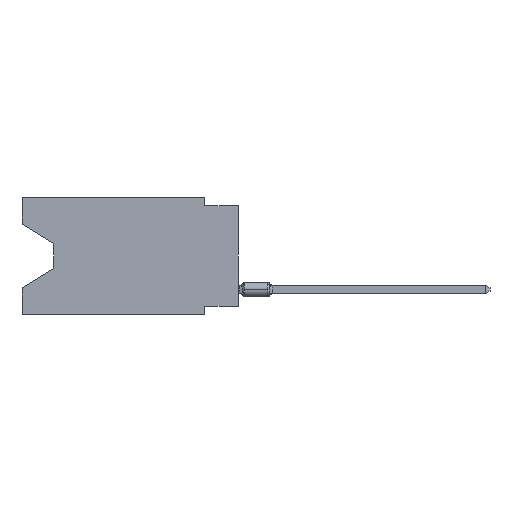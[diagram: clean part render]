
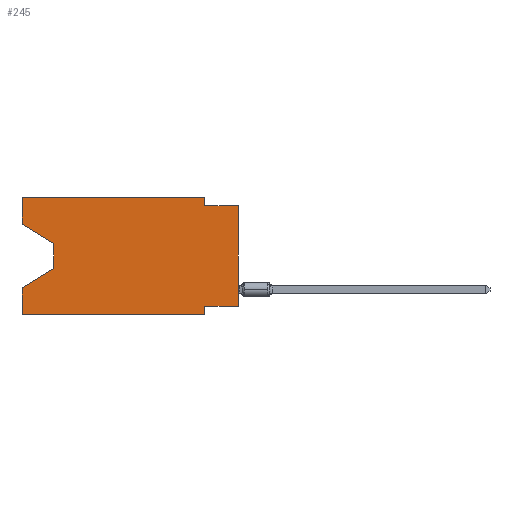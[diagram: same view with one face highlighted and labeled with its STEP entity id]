
A CAD part, left-side view. The second image highlights one B-rep face of the part: STEP entity #245.
In plain terms, the highlighted planar face has unit normal (-1, 0, 0).
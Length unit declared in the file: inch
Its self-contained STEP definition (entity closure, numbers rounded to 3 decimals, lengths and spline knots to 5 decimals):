
#217 = VERTEX_POINT ( 'NONE', #4701 ) ;
#245 = ADVANCED_FACE ( 'NONE', ( #24458 ), #6535, .F. ) ;
#332 = CARTESIAN_POINT ( 'NONE',  ( 0., 0.55, -0.212 ) ) ;
#547 = DIRECTION ( 'NONE',  ( 0., 0., -1. ) ) ;
#1364 = VECTOR ( 'NONE', #547, 39.37008 ) ;
#2369 = DIRECTION ( 'NONE',  ( 0., 0., -1. ) ) ;
#2490 = CARTESIAN_POINT ( 'NONE',  ( 0., 0.1, 0. ) ) ;
#2814 = CARTESIAN_POINT ( 'NONE',  ( 0., 0.645, -0.08025 ) ) ;
#3760 = ORIENTED_EDGE ( 'NONE', *, *, #13887, .T. ) ;
#3884 = LINE ( 'NONE', #23644, #7617 ) ;
#4409 = LINE ( 'NONE', #12259, #15118 ) ;
#4701 = CARTESIAN_POINT ( 'NONE',  ( 0., 0.1, -0.025 ) ) ;
#5200 = LINE ( 'NONE', #8858, #8436 ) ;
#5216 = ORIENTED_EDGE ( 'NONE', *, *, #17313, .F. ) ;
#5710 = DIRECTION ( 'NONE',  ( 0., -1., 0. ) ) ;
#6052 = DIRECTION ( 'NONE',  ( 0., 0., 1. ) ) ;
#6139 = CARTESIAN_POINT ( 'NONE',  ( 0., 0.55, -0.138 ) ) ;
#6485 = VERTEX_POINT ( 'NONE', #6589 ) ;
#6535 = PLANE ( 'NONE',  #13094 ) ;
#6589 = CARTESIAN_POINT ( 'NONE',  ( 0., 0.1, -0.35 ) ) ;
#6834 = VERTEX_POINT ( 'NONE', #2490 ) ;
#7025 = LINE ( 'NONE', #16592, #18294 ) ;
#7617 = VECTOR ( 'NONE', #5710, 39.37008 ) ;
#7631 = VERTEX_POINT ( 'NONE', #20921 ) ;
#7805 = DIRECTION ( 'NONE',  ( 0., 1., 0. ) ) ;
#8436 = VECTOR ( 'NONE', #18684, 39.37008 ) ;
#8643 = VECTOR ( 'NONE', #2369, 39.37008 ) ;
#8858 = CARTESIAN_POINT ( 'NONE',  ( 0., 0.645, 0. ) ) ;
#8985 = CARTESIAN_POINT ( 'NONE',  ( 0., 0.645, 0. ) ) ;
#9284 = EDGE_CURVE ( 'NONE', #16652, #6485, #23923, .T. ) ;
#9373 = ORIENTED_EDGE ( 'NONE', *, *, #17499, .T. ) ;
#9759 = CARTESIAN_POINT ( 'NONE',  ( 0., 0., -0.325 ) ) ;
#9935 = LINE ( 'NONE', #20303, #8643 ) ;
#10164 = CARTESIAN_POINT ( 'NONE',  ( 0., 0.645, -0.35 ) ) ;
#10638 = ORIENTED_EDGE ( 'NONE', *, *, #12898, .F. ) ;
#11161 = ORIENTED_EDGE ( 'NONE', *, *, #24345, .F. ) ;
#11797 = VERTEX_POINT ( 'NONE', #6139 ) ;
#11933 = EDGE_CURVE ( 'NONE', #16652, #7631, #5200, .T. ) ;
#12009 = EDGE_CURVE ( 'NONE', #25308, #6834, #3884, .T. ) ;
#12259 = CARTESIAN_POINT ( 'NONE',  ( 0., 0., 0. ) ) ;
#12898 = EDGE_CURVE ( 'NONE', #15807, #25308, #20046, .T. ) ;
#13094 = AXIS2_PLACEMENT_3D ( 'NONE', #20532, #20670, #14632 ) ;
#13154 = LINE ( 'NONE', #2814, #22991 ) ;
#13517 = VECTOR ( 'NONE', #22338, 39.37008 ) ;
#13703 = LINE ( 'NONE', #9759, #16769 ) ;
#13887 = EDGE_CURVE ( 'NONE', #15807, #11797, #13154, .T. ) ;
#14145 = ORIENTED_EDGE ( 'NONE', *, *, #17354, .F. ) ;
#14245 = DIRECTION ( 'NONE',  ( 0., -1., 0. ) ) ;
#14297 = DIRECTION ( 'NONE',  ( 0., -1., 0. ) ) ;
#14357 = LINE ( 'NONE', #22453, #13517 ) ;
#14573 = ORIENTED_EDGE ( 'NONE', *, *, #11933, .F. ) ;
#14632 = DIRECTION ( 'NONE',  ( 0., 0., -1. ) ) ;
#15118 = VECTOR ( 'NONE', #15911, 39.37008 ) ;
#15290 = ORIENTED_EDGE ( 'NONE', *, *, #23583, .T. ) ;
#15747 = EDGE_CURVE ( 'NONE', #11797, #22293, #16263, .T. ) ;
#15807 = VERTEX_POINT ( 'NONE', #20569 ) ;
#15911 = DIRECTION ( 'NONE',  ( 0., 0., 1. ) ) ;
#16263 = LINE ( 'NONE', #24106, #1364 ) ;
#16431 = VECTOR ( 'NONE', #6052, 39.37008 ) ;
#16592 = CARTESIAN_POINT ( 'NONE',  ( 0., 0.1, 0. ) ) ;
#16652 = VERTEX_POINT ( 'NONE', #10164 ) ;
#16745 = CARTESIAN_POINT ( 'NONE',  ( 0., 0., -0.025 ) ) ;
#16769 = VECTOR ( 'NONE', #7805, 39.37008 ) ;
#16840 = ORIENTED_EDGE ( 'NONE', *, *, #15747, .T. ) ;
#17313 = EDGE_CURVE ( 'NONE', #217, #17632, #24226, .T. ) ;
#17354 = EDGE_CURVE ( 'NONE', #24927, #23276, #13703, .T. ) ;
#17499 = EDGE_CURVE ( 'NONE', #24927, #17632, #4409, .T. ) ;
#17632 = VERTEX_POINT ( 'NONE', #19050 ) ;
#17650 = ORIENTED_EDGE ( 'NONE', *, *, #25441, .F. ) ;
#18294 = VECTOR ( 'NONE', #20521, 39.37008 ) ;
#18684 = DIRECTION ( 'NONE',  ( 0., 0., 1. ) ) ;
#19050 = CARTESIAN_POINT ( 'NONE',  ( 0., 0., -0.025 ) ) ;
#20046 = LINE ( 'NONE', #22015, #16431 ) ;
#20303 = CARTESIAN_POINT ( 'NONE',  ( 0., 0.1, -0.35 ) ) ;
#20521 = DIRECTION ( 'NONE',  ( 0., 0., -1. ) ) ;
#20532 = CARTESIAN_POINT ( 'NONE',  ( 0., 0.645, 0. ) ) ;
#20547 = VECTOR ( 'NONE', #14245, 39.37008 ) ;
#20569 = CARTESIAN_POINT ( 'NONE',  ( 0., 0.645, -0.08025 ) ) ;
#20670 = DIRECTION ( 'NONE',  ( 1., 0., 0. ) ) ;
#20876 = DIRECTION ( 'NONE',  ( 0., -0.855, -0.519 ) ) ;
#20916 = EDGE_LOOP ( 'NONE', ( #3760, #16840, #15290, #14573, #22565, #11161, #14145, #9373, #5216, #17650, #22688, #10638 ) ) ;
#20921 = CARTESIAN_POINT ( 'NONE',  ( 0., 0.645, -0.26975 ) ) ;
#21284 = CARTESIAN_POINT ( 'NONE',  ( 0., 0.1, -0.325 ) ) ;
#22015 = CARTESIAN_POINT ( 'NONE',  ( 0., 0.645, 0. ) ) ;
#22293 = VERTEX_POINT ( 'NONE', #332 ) ;
#22338 = DIRECTION ( 'NONE',  ( 0., 0.855, -0.519 ) ) ;
#22453 = CARTESIAN_POINT ( 'NONE',  ( 0., 0.55, -0.212 ) ) ;
#22565 = ORIENTED_EDGE ( 'NONE', *, *, #9284, .T. ) ;
#22688 = ORIENTED_EDGE ( 'NONE', *, *, #12009, .F. ) ;
#22991 = VECTOR ( 'NONE', #20876, 39.37008 ) ;
#23276 = VERTEX_POINT ( 'NONE', #21284 ) ;
#23583 = EDGE_CURVE ( 'NONE', #22293, #7631, #14357, .T. ) ;
#23644 = CARTESIAN_POINT ( 'NONE',  ( 0., 0.645, 0. ) ) ;
#23923 = LINE ( 'NONE', #24312, #20547 ) ;
#24106 = CARTESIAN_POINT ( 'NONE',  ( 0., 0.55, -0.138 ) ) ;
#24226 = LINE ( 'NONE', #16745, #25545 ) ;
#24312 = CARTESIAN_POINT ( 'NONE',  ( 0., 0.645, -0.35 ) ) ;
#24345 = EDGE_CURVE ( 'NONE', #23276, #6485, #9935, .T. ) ;
#24360 = CARTESIAN_POINT ( 'NONE',  ( 0., 0., -0.325 ) ) ;
#24458 = FACE_OUTER_BOUND ( 'NONE', #20916, .T. ) ;
#24927 = VERTEX_POINT ( 'NONE', #24360 ) ;
#25308 = VERTEX_POINT ( 'NONE', #8985 ) ;
#25441 = EDGE_CURVE ( 'NONE', #6834, #217, #7025, .T. ) ;
#25545 = VECTOR ( 'NONE', #14297, 39.37008 ) ;
